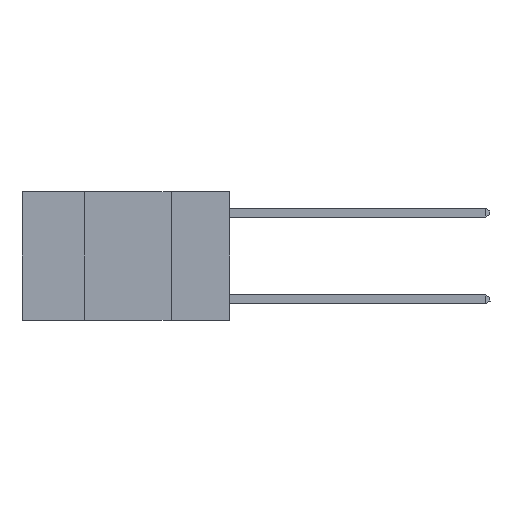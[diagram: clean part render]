
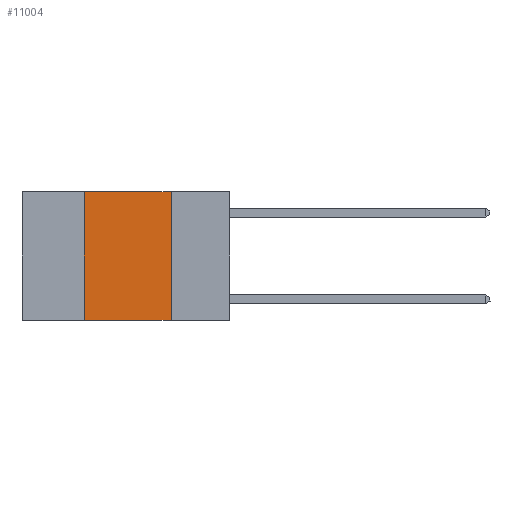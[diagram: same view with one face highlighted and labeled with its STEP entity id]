
A CAD part, left-side view. The second image highlights one B-rep face of the part: STEP entity #11004.
In plain terms, the highlighted planar face has unit normal (-1, 0, 0).
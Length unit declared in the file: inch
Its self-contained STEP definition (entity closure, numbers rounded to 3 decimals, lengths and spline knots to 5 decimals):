
#712 = VERTEX_POINT ( 'NONE', #7523 ) ;
#983 = EDGE_LOOP ( 'NONE', ( #13931, #17289, #18797, #18115 ) ) ;
#1083 = EDGE_CURVE ( 'NONE', #13486, #1462, #12769, .T. ) ;
#1462 = VERTEX_POINT ( 'NONE', #3758 ) ;
#2453 = CARTESIAN_POINT ( 'NONE',  ( 0., 0.6, 0. ) ) ;
#2534 = LINE ( 'NONE', #17717, #17423 ) ;
#3388 = DIRECTION ( 'NONE',  ( 0., 0., -1. ) ) ;
#3758 = CARTESIAN_POINT ( 'NONE',  ( 0., 0.17, 0. ) ) ;
#3991 = PLANE ( 'NONE',  #17863 ) ;
#6972 = DIRECTION ( 'NONE',  ( 0., 0., -1. ) ) ;
#7370 = EDGE_CURVE ( 'NONE', #12386, #712, #2534, .T. ) ;
#7523 = CARTESIAN_POINT ( 'NONE',  ( 0., 0.17, -0.37 ) ) ;
#9849 = LINE ( 'NONE', #12978, #16324 ) ;
#10399 = DIRECTION ( 'NONE',  ( 0., -1., 0. ) ) ;
#10877 = CARTESIAN_POINT ( 'NONE',  ( 0., 0.17, 0. ) ) ;
#11004 = ADVANCED_FACE ( 'NONE', ( #17088 ), #3991, .F. ) ;
#11388 = VECTOR ( 'NONE', #3388, 39.37008 ) ;
#12386 = VERTEX_POINT ( 'NONE', #17370 ) ;
#12769 = LINE ( 'NONE', #13758, #17120 ) ;
#12857 = CARTESIAN_POINT ( 'NONE',  ( 0., 0.42, 0. ) ) ;
#12978 = CARTESIAN_POINT ( 'NONE',  ( 0., 0.42, 0. ) ) ;
#13267 = EDGE_CURVE ( 'NONE', #1462, #712, #15750, .T. ) ;
#13447 = DIRECTION ( 'NONE',  ( 0., -1., 0. ) ) ;
#13486 = VERTEX_POINT ( 'NONE', #12857 ) ;
#13758 = CARTESIAN_POINT ( 'NONE',  ( 0., 0.6, 0. ) ) ;
#13931 = ORIENTED_EDGE ( 'NONE', *, *, #13267, .F. ) ;
#15750 = LINE ( 'NONE', #10877, #11388 ) ;
#15896 = DIRECTION ( 'NONE',  ( 1., 0., 0. ) ) ;
#15928 = DIRECTION ( 'NONE',  ( 0., 0., 1. ) ) ;
#16324 = VECTOR ( 'NONE', #15928, 39.37008 ) ;
#16733 = EDGE_CURVE ( 'NONE', #12386, #13486, #9849, .T. ) ;
#17088 = FACE_OUTER_BOUND ( 'NONE', #983, .T. ) ;
#17120 = VECTOR ( 'NONE', #13447, 39.37008 ) ;
#17289 = ORIENTED_EDGE ( 'NONE', *, *, #1083, .F. ) ;
#17370 = CARTESIAN_POINT ( 'NONE',  ( 0., 0.42, -0.37 ) ) ;
#17423 = VECTOR ( 'NONE', #10399, 39.37008 ) ;
#17717 = CARTESIAN_POINT ( 'NONE',  ( 0., 0.6, -0.37 ) ) ;
#17863 = AXIS2_PLACEMENT_3D ( 'NONE', #2453, #15896, #6972 ) ;
#18115 = ORIENTED_EDGE ( 'NONE', *, *, #7370, .T. ) ;
#18797 = ORIENTED_EDGE ( 'NONE', *, *, #16733, .F. ) ;
